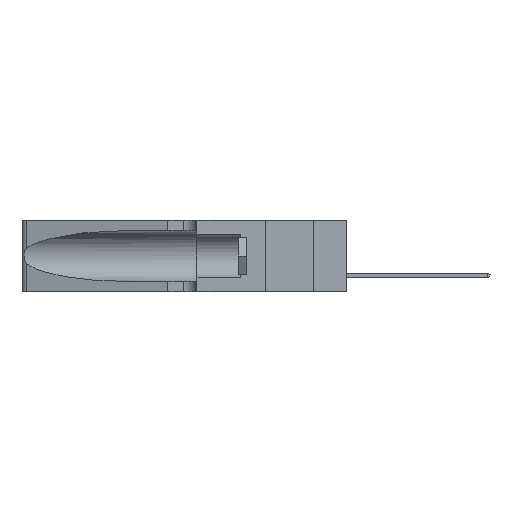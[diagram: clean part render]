
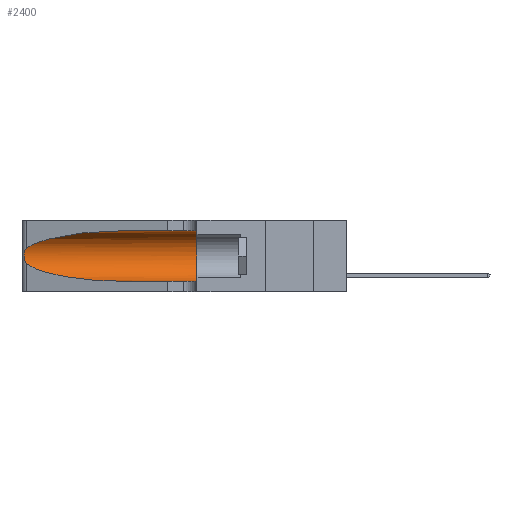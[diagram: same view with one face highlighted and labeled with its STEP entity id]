
A CAD part, left-side view. The second image highlights one B-rep face of the part: STEP entity #2400.
In plain terms, the highlighted cylindrical face has radius 3.308 mm (diameter 6.617 mm), a partial arc.
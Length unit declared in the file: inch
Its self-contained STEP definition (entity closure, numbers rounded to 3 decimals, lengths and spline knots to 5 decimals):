
#352 = EDGE_CURVE ( 'NONE', #7858, #3227, #19356, .T. ) ;
#732 = CARTESIAN_POINT ( 'NONE',  ( 0.26075, 1.23896, 0.178 ) ) ;
#776 = CARTESIAN_POINT ( 'NONE',  ( 0.26075, 1.23896, 0.19203 ) ) ;
#832 = CARTESIAN_POINT ( 'NONE',  ( 0.25555, 1.22993, 0.14849 ) ) ;
#1157 = ORIENTED_EDGE ( 'NONE', *, *, #13010, .T. ) ;
#1351 = FACE_OUTER_BOUND ( 'NONE', #23000, .T. ) ;
#1540 = CARTESIAN_POINT ( 'NONE',  ( 0.1305, 0.35, 0.185 ) ) ;
#2094 = CARTESIAN_POINT ( 'NONE',  ( 0.1305, 0.35, 0.05475 ) ) ;
#2400 = ADVANCED_FACE ( 'NONE', ( #1351 ), #17292, .F. ) ;
#3227 = VERTEX_POINT ( 'NONE', #26601 ) ;
#3307 = CARTESIAN_POINT ( 'NONE',  ( 0.2373, 1.15595, 0.28018 ) ) ;
#3466 =( BOUNDED_CURVE ( )  B_SPLINE_CURVE ( 3, ( #28242, #15296, #30956, #15412 ),
 .UNSPECIFIED., .F., .F. ) 
 B_SPLINE_CURVE_WITH_KNOTS ( ( 4, 4 ),
 ( 3.44316, 4.71239 ),
 .UNSPECIFIED. ) 
 CURVE ( )  GEOMETRIC_REPRESENTATION_ITEM ( )  RATIONAL_B_SPLINE_CURVE ( ( 1., 0.87, 0.87, 1. ) ) 
 REPRESENTATION_ITEM ( '' )  );
#4397 = CARTESIAN_POINT ( 'NONE',  ( 0.25789, 1.23486, 0.15765 ) ) ;
#4657 = DIRECTION ( 'NONE',  ( 0., 0., -1. ) ) ;
#4692 = ORIENTED_EDGE ( 'NONE', *, *, #11190, .T. ) ;
#5022 = CARTESIAN_POINT ( 'NONE',  ( 0.1305, 0.72297, 0.05475 ) ) ;
#5352 = CARTESIAN_POINT ( 'NONE',  ( 0.25487, 1.22718, 0.22369 ) ) ;
#5584 = ORIENTED_EDGE ( 'NONE', *, *, #352, .F. ) ;
#5982 = CARTESIAN_POINT ( 'NONE',  ( 0.25487, 1.22718, 0.14631 ) ) ;
#6083 = CARTESIAN_POINT ( 'NONE',  ( 0.25487, 1.22718, 0.22369 ) ) ;
#7858 = VERTEX_POINT ( 'NONE', #32634 ) ;
#8038 = CARTESIAN_POINT ( 'NONE',  ( 0.1305, 1.61858, 0.31525 ) ) ;
#8455 = VECTOR ( 'NONE', #15147, 39.37008 ) ;
#9011 = VERTEX_POINT ( 'NONE', #2094 ) ;
#9533 =( BOUNDED_CURVE ( )  B_SPLINE_CURVE ( 3, ( #24335, #23862, #3307, #16625 ),
 .UNSPECIFIED., .F., .T. ) 
 B_SPLINE_CURVE_WITH_KNOTS ( ( 4, 4 ),
 ( 1.5708, 2.84003 ),
 .UNSPECIFIED. ) 
 CURVE ( )  GEOMETRIC_REPRESENTATION_ITEM ( )  RATIONAL_B_SPLINE_CURVE ( ( 1., 0.87, 0.87, 1. ) ) 
 REPRESENTATION_ITEM ( '' )  );
#10811 = ORIENTED_EDGE ( 'NONE', *, *, #25805, .T. ) ;
#11190 = EDGE_CURVE ( 'NONE', #7858, #11754, #9533, .T. ) ;
#11754 = VERTEX_POINT ( 'NONE', #5352 ) ;
#11902 = EDGE_CURVE ( 'NONE', #11754, #26782, #13635, .T. ) ;
#13010 = EDGE_CURVE ( 'NONE', #26782, #25788, #3466, .T. ) ;
#13097 = AXIS2_PLACEMENT_3D ( 'NONE', #25341, #14514, #4657 ) ;
#13635 = B_SPLINE_CURVE_WITH_KNOTS ( 'NONE', 3,
 ( #6083, #31964, #32294, #26947, #16849, #26722, #776, #732, #23843, #31690, #4397, #14244, #832, #27172 ),
 .UNSPECIFIED., .F., .F.,
 ( 4, 2, 2, 2, 2, 2, 4 ),
 ( 0., 0.00027, 0.00053, 0.00107, 0.0016, 0.00187, 0.00214 ),
 .UNSPECIFIED. ) ;
#14244 = CARTESIAN_POINT ( 'NONE',  ( 0.25639, 1.23186, 0.15144 ) ) ;
#14497 = ORIENTED_EDGE ( 'NONE', *, *, #25137, .F. ) ;
#14514 = DIRECTION ( 'NONE',  ( 0., -1., 0. ) ) ;
#15147 = DIRECTION ( 'NONE',  ( 0., -1., 0. ) ) ;
#15296 = CARTESIAN_POINT ( 'NONE',  ( 0.2373, 1.15595, 0.08982 ) ) ;
#15394 = LINE ( 'NONE', #31038, #8455 ) ;
#15412 = CARTESIAN_POINT ( 'NONE',  ( 0.1305, 0.72297, 0.05475 ) ) ;
#16625 = CARTESIAN_POINT ( 'NONE',  ( 0.25487, 1.22718, 0.22369 ) ) ;
#16849 = CARTESIAN_POINT ( 'NONE',  ( 0.25854, 1.2359, 0.20912 ) ) ;
#17292 = CYLINDRICAL_SURFACE ( 'NONE', #13097, 0.13025 ) ;
#17383 = VECTOR ( 'NONE', #26159, 39.37008 ) ;
#19356 = LINE ( 'NONE', #8038, #17383 ) ;
#19503 = DIRECTION ( 'NONE',  ( 0., 0., 1. ) ) ;
#23000 = EDGE_LOOP ( 'NONE', ( #4692, #25892, #1157, #10811, #14497, #5584 ) ) ;
#23843 = CARTESIAN_POINT ( 'NONE',  ( 0.26017, 1.23833, 0.17102 ) ) ;
#23862 = CARTESIAN_POINT ( 'NONE',  ( 0.18966, 0.96281, 0.31525 ) ) ;
#24335 = CARTESIAN_POINT ( 'NONE',  ( 0.1305, 0.72297, 0.31525 ) ) ;
#25137 = EDGE_CURVE ( 'NONE', #3227, #9011, #28454, .T. ) ;
#25341 = CARTESIAN_POINT ( 'NONE',  ( 0.1305, 1.61858, 0.185 ) ) ;
#25788 = VERTEX_POINT ( 'NONE', #5022 ) ;
#25805 = EDGE_CURVE ( 'NONE', #25788, #9011, #15394, .T. ) ;
#25892 = ORIENTED_EDGE ( 'NONE', *, *, #11902, .T. ) ;
#26159 = DIRECTION ( 'NONE',  ( 0., -1., 0. ) ) ;
#26601 = CARTESIAN_POINT ( 'NONE',  ( 0.1305, 0.35, 0.31525 ) ) ;
#26722 = CARTESIAN_POINT ( 'NONE',  ( 0.26018, 1.23835, 0.19895 ) ) ;
#26782 = VERTEX_POINT ( 'NONE', #5982 ) ;
#26947 = CARTESIAN_POINT ( 'NONE',  ( 0.25787, 1.23484, 0.2124 ) ) ;
#27172 = CARTESIAN_POINT ( 'NONE',  ( 0.25487, 1.22718, 0.14631 ) ) ;
#27703 = DIRECTION ( 'NONE',  ( 0., 1., 0. ) ) ;
#28242 = CARTESIAN_POINT ( 'NONE',  ( 0.25487, 1.22718, 0.14631 ) ) ;
#28454 = CIRCLE ( 'NONE', #30587, 0.13025 ) ;
#30587 = AXIS2_PLACEMENT_3D ( 'NONE', #1540, #27703, #19503 ) ;
#30956 = CARTESIAN_POINT ( 'NONE',  ( 0.18966, 0.96281, 0.05475 ) ) ;
#31038 = CARTESIAN_POINT ( 'NONE',  ( 0.1305, 1.61858, 0.05475 ) ) ;
#31690 = CARTESIAN_POINT ( 'NONE',  ( 0.25856, 1.23593, 0.16098 ) ) ;
#31964 = CARTESIAN_POINT ( 'NONE',  ( 0.25555, 1.22994, 0.2215 ) ) ;
#32294 = CARTESIAN_POINT ( 'NONE',  ( 0.25639, 1.23184, 0.21858 ) ) ;
#32634 = CARTESIAN_POINT ( 'NONE',  ( 0.1305, 0.72297, 0.31525 ) ) ;
